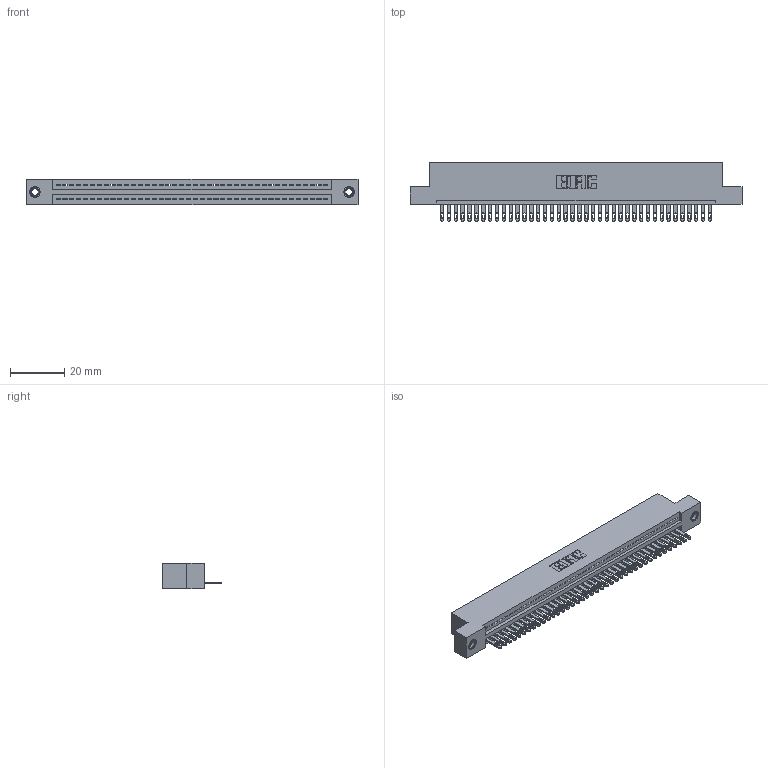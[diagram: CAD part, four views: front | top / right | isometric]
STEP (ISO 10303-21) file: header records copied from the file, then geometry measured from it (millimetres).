
FILE_DESCRIPTION (( 'STEP AP203' ), '1' );
FILE_NAME ('895-040-500-107.STEP', '2020-09-26T02:49:24', ( '' ), ( '' ), 'SwSTEP 2.0', 'SolidWorks 2020', '' );
FILE_SCHEMA (( 'CONFIG_CONTROL_DESIGN' ));
Length unit declared in the file: inch
Products named in the file (4): 345-250-001_345-250-005-103; 895-040-500-107; 345-292-001_345-293-100; 845 Part_Flush Mounting Lugs - 0.156 Dia-TI
Assembly tree (43 placements, depth 2):
  895-040-500-107
    845 Part_Flush Mounting Lugs - 0.156 Dia-TI
    345-292-001_345-293-100  x40
    345-250-001_345-250-005-103  x2
Bounding box: 122.81 x 21.51 x 9.4 mm (x, y, z)
Volume: 11659.4 mm3; surface area: 15589.5 mm2
Topology: 43 solids, 43 shells, 2346 faces, 7197 edges, 4790 vertices
Faces by surface type: plane 1472, cylinder 858, cone 12, torus 4
Entity records: 31490 total; most frequent: CARTESIAN_POINT 5435, ORIENTED_EDGE 5402, DIRECTION 4779, EDGE_CURVE 2701, LINE 2385, VECTOR 2385, VERTEX_POINT 1796, AXIS2_PLACEMENT_3D 1197
